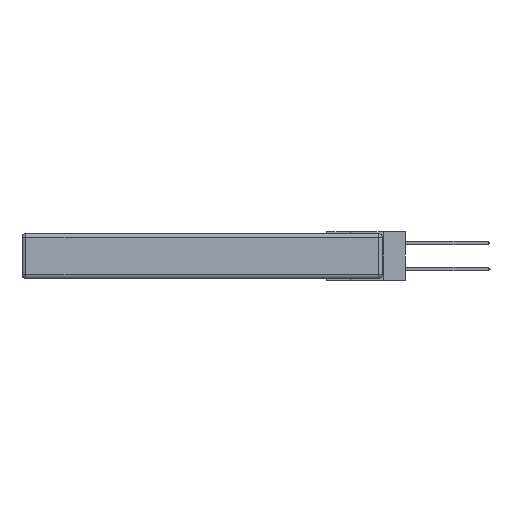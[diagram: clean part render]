
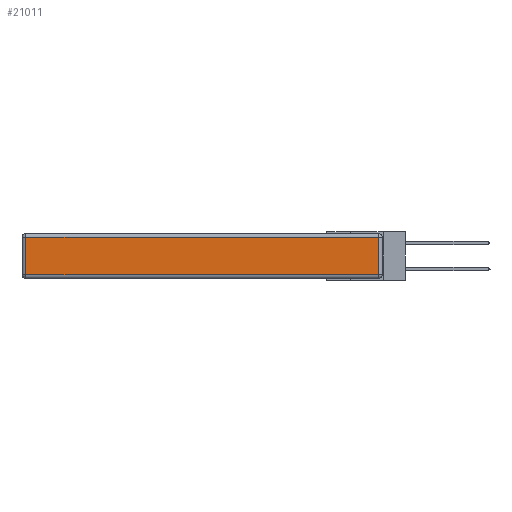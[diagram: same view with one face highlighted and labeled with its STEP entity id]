
A CAD part, left-side view. The second image highlights one B-rep face of the part: STEP entity #21011.
In plain terms, the highlighted planar face has unit normal (-1, 0, 0).
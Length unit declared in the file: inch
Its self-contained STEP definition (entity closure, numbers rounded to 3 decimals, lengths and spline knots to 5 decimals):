
#752 = VECTOR ( 'NONE', #24084, 39.37008 ) ;
#1004 = VERTEX_POINT ( 'NONE', #21928 ) ;
#2739 = CARTESIAN_POINT ( 'NONE',  ( 0., 2.72, -0.313 ) ) ;
#3674 = VECTOR ( 'NONE', #30236, 39.37008 ) ;
#3985 = CARTESIAN_POINT ( 'NONE',  ( 0., 0.03, -0.313 ) ) ;
#5072 = VECTOR ( 'NONE', #34393, 39.37008 ) ;
#6303 = VECTOR ( 'NONE', #17647, 39.37008 ) ;
#6541 = CARTESIAN_POINT ( 'NONE',  ( 0., 2.75, -0.03 ) ) ;
#7178 = LINE ( 'NONE', #6541, #6303 ) ;
#7562 = EDGE_CURVE ( 'NONE', #1004, #33101, #7178, .T. ) ;
#12395 = EDGE_CURVE ( 'NONE', #33101, #28831, #34795, .T. ) ;
#12672 = EDGE_CURVE ( 'NONE', #28831, #35565, #20313, .T. ) ;
#13233 = ORIENTED_EDGE ( 'NONE', *, *, #12672, .T. ) ;
#13684 = LINE ( 'NONE', #21599, #3674 ) ;
#15125 = CARTESIAN_POINT ( 'NONE',  ( 0., 0., -0.343 ) ) ;
#16571 = ORIENTED_EDGE ( 'NONE', *, *, #12395, .T. ) ;
#17581 = DIRECTION ( 'NONE',  ( -1., 0., 0. ) ) ;
#17647 = DIRECTION ( 'NONE',  ( 0., 1., 0. ) ) ;
#18919 = FACE_OUTER_BOUND ( 'NONE', #19368, .T. ) ;
#19368 = EDGE_LOOP ( 'NONE', ( #13233, #21686, #22549, #16571 ) ) ;
#19461 = CARTESIAN_POINT ( 'NONE',  ( 0., 2.72, -0.03 ) ) ;
#20270 = PLANE ( 'NONE',  #21742 ) ;
#20313 = LINE ( 'NONE', #21614, #752 ) ;
#21011 = ADVANCED_FACE ( 'NONE', ( #18919 ), #20270, .T. ) ;
#21599 = CARTESIAN_POINT ( 'NONE',  ( 0., 0.03, -0.343 ) ) ;
#21614 = CARTESIAN_POINT ( 'NONE',  ( 0., 0., -0.313 ) ) ;
#21686 = ORIENTED_EDGE ( 'NONE', *, *, #23697, .T. ) ;
#21742 = AXIS2_PLACEMENT_3D ( 'NONE', #15125, #17581, #34360 ) ;
#21928 = CARTESIAN_POINT ( 'NONE',  ( 0., 0.03, -0.03 ) ) ;
#22549 = ORIENTED_EDGE ( 'NONE', *, *, #7562, .T. ) ;
#23697 = EDGE_CURVE ( 'NONE', #35565, #1004, #13684, .T. ) ;
#24084 = DIRECTION ( 'NONE',  ( 0., -1., 0. ) ) ;
#28831 = VERTEX_POINT ( 'NONE', #2739 ) ;
#30236 = DIRECTION ( 'NONE',  ( 0., 0., 1. ) ) ;
#31251 = CARTESIAN_POINT ( 'NONE',  ( 0., 2.72, -0.343 ) ) ;
#33101 = VERTEX_POINT ( 'NONE', #19461 ) ;
#34360 = DIRECTION ( 'NONE',  ( 0., 0., 1. ) ) ;
#34393 = DIRECTION ( 'NONE',  ( 0., 0., -1. ) ) ;
#34795 = LINE ( 'NONE', #31251, #5072 ) ;
#35565 = VERTEX_POINT ( 'NONE', #3985 ) ;
